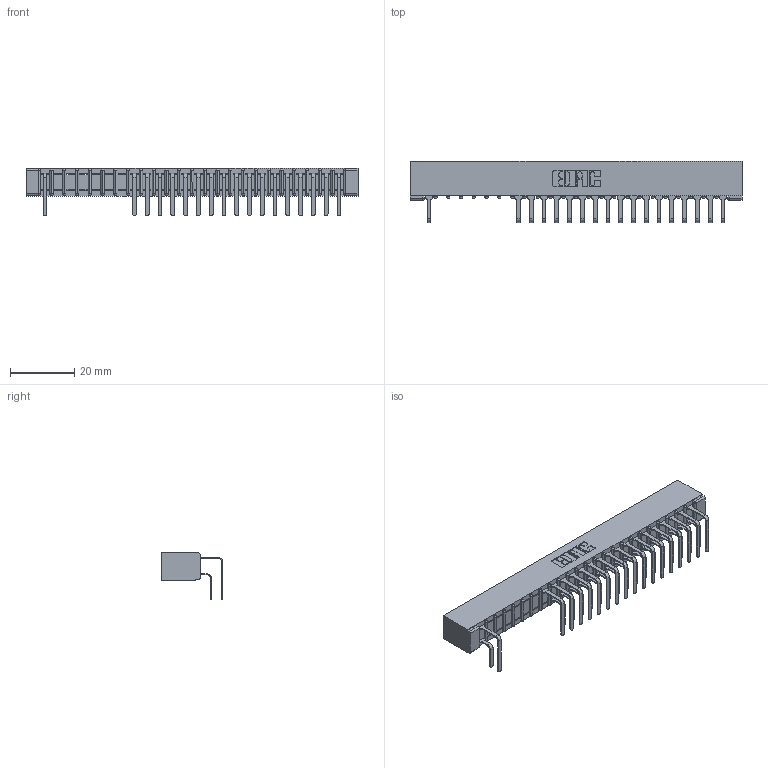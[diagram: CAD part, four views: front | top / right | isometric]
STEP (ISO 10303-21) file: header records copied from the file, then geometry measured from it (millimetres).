
FILE_DESCRIPTION (( 'STEP AP203' ), '1' );
FILE_NAME ('307-048-558-201.STEP', '2018-08-06T04:00:39', ( '' ), ( '' ), 'SwSTEP 2.0', 'SolidWorks 2016', '' );
FILE_SCHEMA (( 'CONFIG_CONTROL_DESIGN' ));
Length unit declared in the file: inch
Products named in the file (4): 307 Part_No Mounting Lugs; 307-290-001_558 559 - 1 (Single); 307-290-001_558 - 2 (Single); 307-048-558-201
Assembly tree (36 placements, depth 2):
  307-048-558-201
    307 Part_No Mounting Lugs
    307-290-001_558 559 - 1 (Single)  x17
    307-290-001_558 - 2 (Single)  x18
Bounding box: 102.97 x 18.96 x 14.81 mm (x, y, z)
Volume: 6956.8 mm3; surface area: 12751.9 mm2
Topology: 36 solids, 36 shells, 2015 faces, 5685 edges, 3674 vertices
Faces by surface type: plane 1299, cylinder 666, sphere 50
Entity records: 24315 total; most frequent: CARTESIAN_POINT 4037, ORIENTED_EDGE 4010, DIRECTION 3947, EDGE_CURVE 2005, VECTOR 1531, LINE 1531, VERTEX_POINT 1298, AXIS2_PLACEMENT_3D 1208
